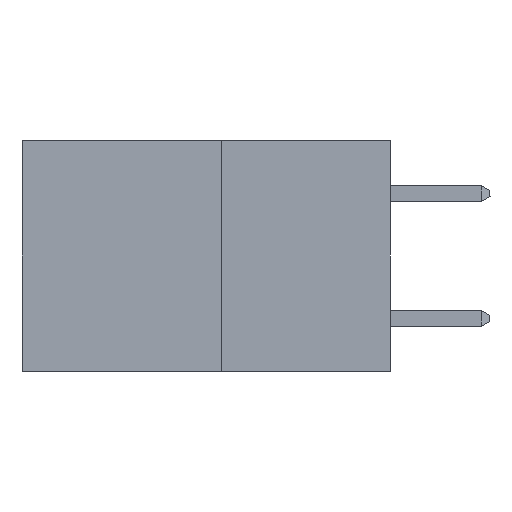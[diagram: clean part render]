
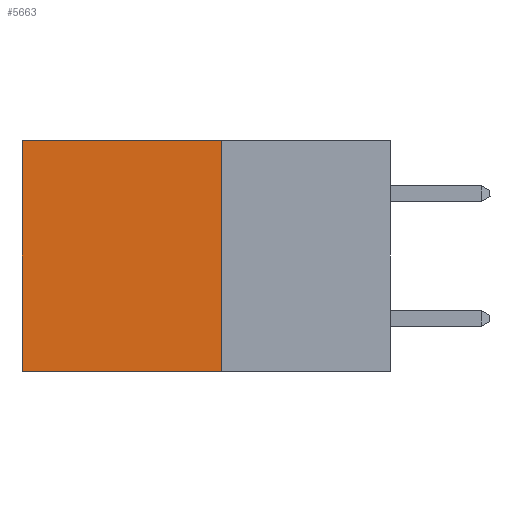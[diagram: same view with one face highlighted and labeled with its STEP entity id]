
A CAD part, left-side view. The second image highlights one B-rep face of the part: STEP entity #5663.
In plain terms, the highlighted planar face has unit normal (-1, 0, 0).
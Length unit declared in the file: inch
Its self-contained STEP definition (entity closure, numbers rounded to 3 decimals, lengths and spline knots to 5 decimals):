
#479 = VECTOR ( 'NONE', #15531, 39.37008 ) ;
#2519 = CARTESIAN_POINT ( 'NONE',  ( 0.277, 0.27, 0. ) ) ;
#2929 = CARTESIAN_POINT ( 'NONE',  ( 0.277, 0.27, -0.37 ) ) ;
#3091 = LINE ( 'NONE', #4622, #11786 ) ;
#3883 = EDGE_CURVE ( 'NONE', #20716, #13409, #8591, .T. ) ;
#4463 = DIRECTION ( 'NONE',  ( 0., 0., -1. ) ) ;
#4501 = ORIENTED_EDGE ( 'NONE', *, *, #12218, .F. ) ;
#4622 = CARTESIAN_POINT ( 'NONE',  ( 0.277, 0.27, -0.37 ) ) ;
#5237 = PLANE ( 'NONE',  #13615 ) ;
#5413 = EDGE_LOOP ( 'NONE', ( #13088, #4501, #19048, #16908 ) ) ;
#5473 = CARTESIAN_POINT ( 'NONE',  ( 0.277, 0.27, -0.37 ) ) ;
#5663 = ADVANCED_FACE ( 'NONE', ( #11509 ), #5237, .F. ) ;
#8059 = DIRECTION ( 'NONE',  ( 0., 1., 0. ) ) ;
#8133 = DIRECTION ( 'NONE',  ( 0., 0., -1. ) ) ;
#8340 = CARTESIAN_POINT ( 'NONE',  ( 0.277, 0.59, 0. ) ) ;
#8591 = LINE ( 'NONE', #15275, #20563 ) ;
#8942 = CARTESIAN_POINT ( 'NONE',  ( 0.277, 0.59, -0.37 ) ) ;
#9244 = LINE ( 'NONE', #8942, #479 ) ;
#11509 = FACE_OUTER_BOUND ( 'NONE', #5413, .T. ) ;
#11786 = VECTOR ( 'NONE', #8133, 39.37008 ) ;
#12218 = EDGE_CURVE ( 'NONE', #18449, #20865, #20194, .T. ) ;
#13088 = ORIENTED_EDGE ( 'NONE', *, *, #17723, .T. ) ;
#13409 = VERTEX_POINT ( 'NONE', #8340 ) ;
#13615 = AXIS2_PLACEMENT_3D ( 'NONE', #5473, #17534, #4463 ) ;
#13671 = EDGE_CURVE ( 'NONE', #20716, #18449, #3091, .T. ) ;
#15209 = DIRECTION ( 'NONE',  ( 0., 1., 0. ) ) ;
#15275 = CARTESIAN_POINT ( 'NONE',  ( 0.277, 0.27, 0. ) ) ;
#15531 = DIRECTION ( 'NONE',  ( 0., 0., -1. ) ) ;
#15580 = CARTESIAN_POINT ( 'NONE',  ( 0.277, 0.27, -0.37 ) ) ;
#16134 = VECTOR ( 'NONE', #8059, 39.37008 ) ;
#16908 = ORIENTED_EDGE ( 'NONE', *, *, #3883, .T. ) ;
#17534 = DIRECTION ( 'NONE',  ( 1., 0., 0. ) ) ;
#17723 = EDGE_CURVE ( 'NONE', #13409, #20865, #9244, .T. ) ;
#18449 = VERTEX_POINT ( 'NONE', #15580 ) ;
#19048 = ORIENTED_EDGE ( 'NONE', *, *, #13671, .F. ) ;
#20194 = LINE ( 'NONE', #2929, #16134 ) ;
#20483 = CARTESIAN_POINT ( 'NONE',  ( 0.277, 0.59, -0.37 ) ) ;
#20563 = VECTOR ( 'NONE', #15209, 39.37008 ) ;
#20716 = VERTEX_POINT ( 'NONE', #2519 ) ;
#20865 = VERTEX_POINT ( 'NONE', #20483 ) ;
